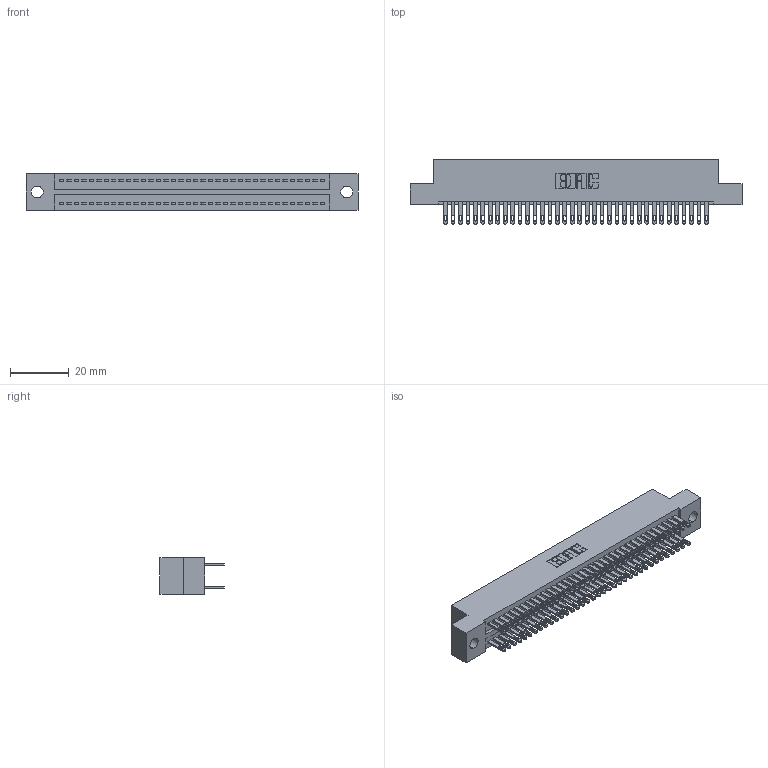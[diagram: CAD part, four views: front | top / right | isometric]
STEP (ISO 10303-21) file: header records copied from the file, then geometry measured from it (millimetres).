
FILE_DESCRIPTION (( 'STEP AP203' ), '1' );
FILE_NAME ('325-072-500-209.STEP', '2020-02-25T03:51:54', ( '' ), ( '' ), 'SwSTEP 2.0', 'SolidWorks 2016', '' );
FILE_SCHEMA (( 'CONFIG_CONTROL_DESIGN' ));
Length unit declared in the file: inch
Products named in the file (3): 325-292-001_325-293-100; 325 Part_.160 TH; 325-072-500-209
Assembly tree (73 placements, depth 2):
  325-072-500-209
    325 Part_.160 TH
    325-292-001_325-293-100  x72
Bounding box: 113.16 x 21.84 x 12.45 mm (x, y, z)
Volume: 14543.5 mm3; surface area: 18133.9 mm2
Topology: 73 solids, 73 shells, 3570 faces, 10895 edges, 7262 vertices
Faces by surface type: plane 2230, cylinder 1340
Entity records: 23869 total; most frequent: CARTESIAN_POINT 3962, ORIENTED_EDGE 3898, DIRECTION 3397, EDGE_CURVE 1949, LINE 1817, VECTOR 1817, VERTEX_POINT 1298, AXIS2_PLACEMENT_3D 790
